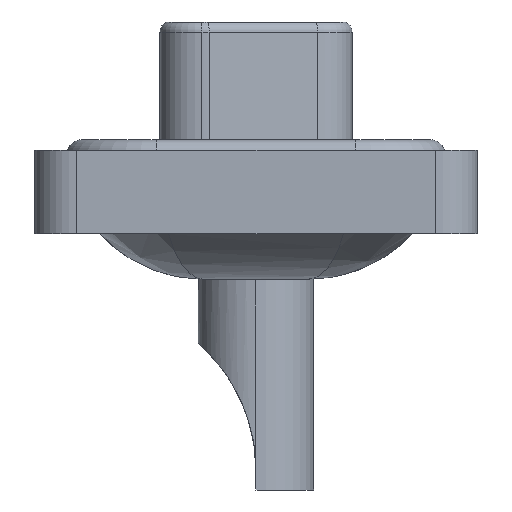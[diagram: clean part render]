
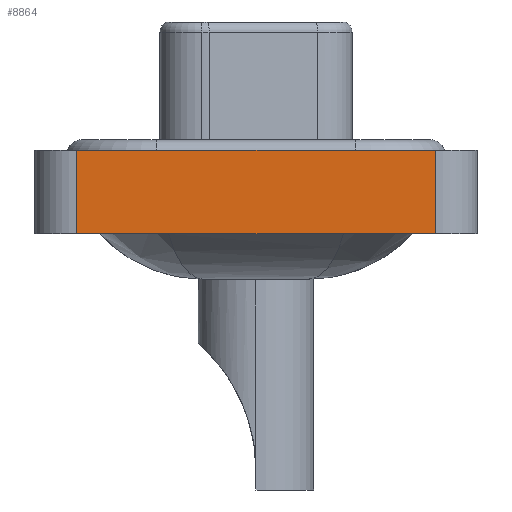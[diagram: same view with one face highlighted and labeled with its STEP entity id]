
A CAD part, left-side view. The second image highlights one B-rep face of the part: STEP entity #8864.
In plain terms, the highlighted planar face has unit normal (-1, 0, 0).
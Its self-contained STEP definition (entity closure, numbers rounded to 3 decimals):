
#792 = VERTEX_POINT ( 'NONE', #12762 ) ;
#794 = LINE ( 'NONE', #13480, #11398 ) ;
#1063 = VECTOR ( 'NONE', #8034, 1000. ) ;
#1749 = LINE ( 'NONE', #6425, #8263 ) ;
#2630 = DIRECTION ( 'NONE',  ( -1., 0., 0. ) ) ;
#2954 = DIRECTION ( 'NONE',  ( 0., -1., 0. ) ) ;
#3111 = CARTESIAN_POINT ( 'NONE',  ( -7.25, 8.55, -3.6 ) ) ;
#3770 = VERTEX_POINT ( 'NONE', #6132 ) ;
#3772 = VERTEX_POINT ( 'NONE', #14284 ) ;
#4012 = ORIENTED_EDGE ( 'NONE', *, *, #8665, .F. ) ;
#4770 = PLANE ( 'NONE',  #5989 ) ;
#5241 = VECTOR ( 'NONE', #7797, 1000. ) ;
#5496 = CARTESIAN_POINT ( 'NONE',  ( -7.25, -8.55, -3.6 ) ) ;
#5624 = CARTESIAN_POINT ( 'NONE',  ( -7.25, 8.55, -3.6 ) ) ;
#5989 = AXIS2_PLACEMENT_3D ( 'NONE', #14150, #2630, #11014 ) ;
#6132 = CARTESIAN_POINT ( 'NONE',  ( -7.25, -8.55, -3.6 ) ) ;
#6425 = CARTESIAN_POINT ( 'NONE',  ( -7.25, -8.55, -3.6 ) ) ;
#6778 = EDGE_CURVE ( 'NONE', #9999, #3770, #11502, .T. ) ;
#7538 = ORIENTED_EDGE ( 'NONE', *, *, #14736, .T. ) ;
#7797 = DIRECTION ( 'NONE',  ( 0., 0., 1. ) ) ;
#7823 = DIRECTION ( 'NONE',  ( 0., 0., 1. ) ) ;
#8034 = DIRECTION ( 'NONE',  ( 0., -1., 0. ) ) ;
#8263 = VECTOR ( 'NONE', #7823, 1000. ) ;
#8665 = EDGE_CURVE ( 'NONE', #792, #3772, #794, .T. ) ;
#8864 = ADVANCED_FACE ( 'NONE', ( #10547 ), #4770, .T. ) ;
#9843 = ORIENTED_EDGE ( 'NONE', *, *, #6778, .T. ) ;
#9999 = VERTEX_POINT ( 'NONE', #5624 ) ;
#10547 = FACE_OUTER_BOUND ( 'NONE', #11003, .T. ) ;
#10593 = EDGE_CURVE ( 'NONE', #9999, #792, #14781, .T. ) ;
#10935 = ORIENTED_EDGE ( 'NONE', *, *, #10593, .F. ) ;
#11003 = EDGE_LOOP ( 'NONE', ( #7538, #4012, #10935, #9843 ) ) ;
#11014 = DIRECTION ( 'NONE',  ( 0., 0., 1. ) ) ;
#11398 = VECTOR ( 'NONE', #2954, 1000. ) ;
#11502 = LINE ( 'NONE', #5496, #1063 ) ;
#12762 = CARTESIAN_POINT ( 'NONE',  ( -7.25, 8.55, 0.4 ) ) ;
#13480 = CARTESIAN_POINT ( 'NONE',  ( -7.25, -8.55, 0.4 ) ) ;
#14150 = CARTESIAN_POINT ( 'NONE',  ( -7.25, -8.55, -3.6 ) ) ;
#14284 = CARTESIAN_POINT ( 'NONE',  ( -7.25, -8.55, 0.4 ) ) ;
#14736 = EDGE_CURVE ( 'NONE', #3770, #3772, #1749, .T. ) ;
#14781 = LINE ( 'NONE', #3111, #5241 ) ;
